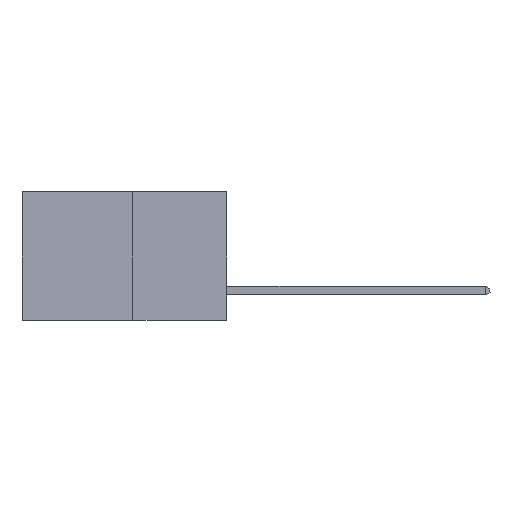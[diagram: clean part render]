
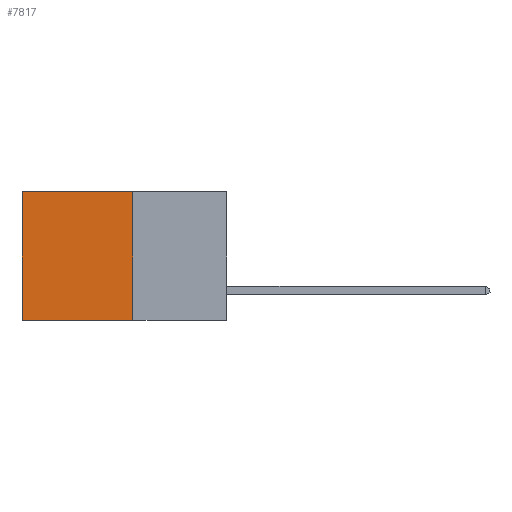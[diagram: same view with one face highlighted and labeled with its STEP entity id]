
A CAD part, left-side view. The second image highlights one B-rep face of the part: STEP entity #7817.
In plain terms, the highlighted planar face has unit normal (-1, 0, 0).
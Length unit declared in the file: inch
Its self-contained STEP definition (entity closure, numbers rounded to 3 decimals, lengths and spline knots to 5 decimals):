
#296 = LINE ( 'NONE', #21045, #16632 ) ;
#396 = AXIS2_PLACEMENT_3D ( 'NONE', #3565, #3470, #3433 ) ;
#1672 = DIRECTION ( 'NONE',  ( 0., 1., 0. ) ) ;
#1776 = CARTESIAN_POINT ( 'NONE',  ( 0.277, 0.27, -0.37 ) ) ;
#2273 = DIRECTION ( 'NONE',  ( 0., 0., -1. ) ) ;
#2516 = EDGE_CURVE ( 'NONE', #4806, #6071, #21766, .T. ) ;
#2767 = ORIENTED_EDGE ( 'NONE', *, *, #6126, .F. ) ;
#3380 = VECTOR ( 'NONE', #2273, 39.37008 ) ;
#3433 = DIRECTION ( 'NONE',  ( 0., 0., -1. ) ) ;
#3470 = DIRECTION ( 'NONE',  ( 1., 0., 0. ) ) ;
#3565 = CARTESIAN_POINT ( 'NONE',  ( 0.277, 0.27, -0.37 ) ) ;
#3566 = PLANE ( 'NONE',  #396 ) ;
#4253 = FACE_OUTER_BOUND ( 'NONE', #13179, .T. ) ;
#4294 = CARTESIAN_POINT ( 'NONE',  ( 0.277, 0.27, -0.37 ) ) ;
#4371 = CARTESIAN_POINT ( 'NONE',  ( 0.277, 0.27, -0.37 ) ) ;
#4637 = LINE ( 'NONE', #15223, #22314 ) ;
#4806 = VERTEX_POINT ( 'NONE', #18463 ) ;
#6071 = VERTEX_POINT ( 'NONE', #4371 ) ;
#6126 = EDGE_CURVE ( 'NONE', #6071, #14396, #20218, .T. ) ;
#6646 = EDGE_CURVE ( 'NONE', #9662, #14396, #296, .T. ) ;
#7817 = ADVANCED_FACE ( 'NONE', ( #4253 ), #3566, .F. ) ;
#8396 = CARTESIAN_POINT ( 'NONE',  ( 0.277, 0.59, -0.37 ) ) ;
#9662 = VERTEX_POINT ( 'NONE', #22099 ) ;
#13179 = EDGE_LOOP ( 'NONE', ( #22047, #2767, #20779, #27665 ) ) ;
#14396 = VERTEX_POINT ( 'NONE', #8396 ) ;
#15223 = CARTESIAN_POINT ( 'NONE',  ( 0.277, 0.27, 0. ) ) ;
#16632 = VECTOR ( 'NONE', #20437, 39.37008 ) ;
#18463 = CARTESIAN_POINT ( 'NONE',  ( 0.277, 0.27, 0. ) ) ;
#19503 = VECTOR ( 'NONE', #1672, 39.37008 ) ;
#20218 = LINE ( 'NONE', #1776, #19503 ) ;
#20437 = DIRECTION ( 'NONE',  ( 0., 0., -1. ) ) ;
#20779 = ORIENTED_EDGE ( 'NONE', *, *, #2516, .F. ) ;
#21045 = CARTESIAN_POINT ( 'NONE',  ( 0.277, 0.59, -0.37 ) ) ;
#21766 = LINE ( 'NONE', #4294, #3380 ) ;
#22047 = ORIENTED_EDGE ( 'NONE', *, *, #6646, .T. ) ;
#22092 = DIRECTION ( 'NONE',  ( 0., 1., 0. ) ) ;
#22099 = CARTESIAN_POINT ( 'NONE',  ( 0.277, 0.59, 0. ) ) ;
#22314 = VECTOR ( 'NONE', #22092, 39.37008 ) ;
#25139 = EDGE_CURVE ( 'NONE', #4806, #9662, #4637, .T. ) ;
#27665 = ORIENTED_EDGE ( 'NONE', *, *, #25139, .T. ) ;
